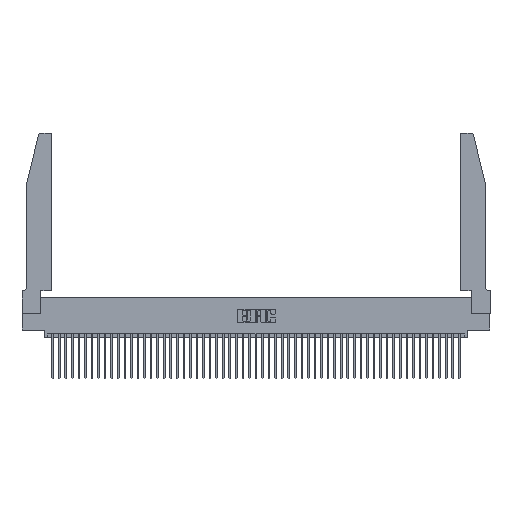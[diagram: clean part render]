
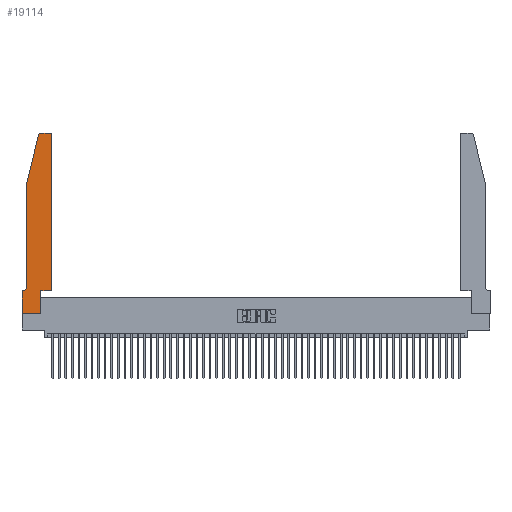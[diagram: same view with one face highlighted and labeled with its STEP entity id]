
A CAD part, top view. The second image highlights one B-rep face of the part: STEP entity #19114.
In plain terms, the highlighted planar face has unit normal (0, 0, 1).
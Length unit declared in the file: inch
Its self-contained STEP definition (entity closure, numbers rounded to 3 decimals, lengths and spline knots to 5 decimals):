
#620 = EDGE_CURVE ( 'NONE', #5873, #29523, #31803, .T. ) ;
#1578 = ORIENTED_EDGE ( 'NONE', *, *, #41890, .T. ) ;
#2566 = VERTEX_POINT ( 'NONE', #39432 ) ;
#3082 = LINE ( 'NONE', #10663, #44157 ) ;
#3701 = CARTESIAN_POINT ( 'NONE',  ( 0.2865, 0.35, 0.37 ) ) ;
#4043 = DIRECTION ( 'NONE',  ( 1., 0., 0. ) ) ;
#4076 = CARTESIAN_POINT ( 'NONE',  ( 0.25487, 2.72718, 0.37 ) ) ;
#4559 = LINE ( 'NONE', #41154, #24607 ) ;
#5214 = DIRECTION ( 'NONE',  ( 0., 0., -1. ) ) ;
#5634 = VERTEX_POINT ( 'NONE', #17853 ) ;
#5873 = VERTEX_POINT ( 'NONE', #9350 ) ;
#6541 = DIRECTION ( 'NONE',  ( 0., -1., 0. ) ) ;
#7667 = VECTOR ( 'NONE', #51362, 39.37008 ) ;
#7882 = DIRECTION ( 'NONE',  ( 0., 1., 0. ) ) ;
#8550 = VERTEX_POINT ( 'NONE', #41912 ) ;
#8673 = LINE ( 'NONE', #29030, #28649 ) ;
#9350 = CARTESIAN_POINT ( 'NONE',  ( 0.0755, 2., 0.37 ) ) ;
#10038 = CARTESIAN_POINT ( 'NONE',  ( 0.4505, 0.35, 0.37 ) ) ;
#10663 = CARTESIAN_POINT ( 'NONE',  ( 0., 0., 0.37 ) ) ;
#10808 = DIRECTION ( 'NONE',  ( 0., -1., 0. ) ) ;
#10912 = EDGE_CURVE ( 'NONE', #2566, #21228, #50021, .T. ) ;
#11011 = CARTESIAN_POINT ( 'NONE',  ( 0.0055, 0.35, 0.37 ) ) ;
#13199 = EDGE_LOOP ( 'NONE', ( #32097, #46073, #20815, #49589, #14871, #13841, #31570, #37342, #35025, #29976, #1578, #30749 ) ) ;
#13446 = CIRCLE ( 'NONE', #44620, 0.03 ) ;
#13841 = ORIENTED_EDGE ( 'NONE', *, *, #39261, .T. ) ;
#13898 = DIRECTION ( 'NONE',  ( 0., 0., 1. ) ) ;
#14679 = CARTESIAN_POINT ( 'NONE',  ( 0.284, 2.75, 0.37 ) ) ;
#14871 = ORIENTED_EDGE ( 'NONE', *, *, #26677, .T. ) ;
#14965 = PLANE ( 'NONE',  #31981 ) ;
#15137 = DIRECTION ( 'NONE',  ( 1., 0., 0. ) ) ;
#15198 = CIRCLE ( 'NONE', #34044, 0.03 ) ;
#17115 = LINE ( 'NONE', #49253, #26450 ) ;
#17155 = VECTOR ( 'NONE', #7882, 39.37008 ) ;
#17853 = CARTESIAN_POINT ( 'NONE',  ( 0.4505, 2.72, 0.37 ) ) ;
#18356 = LINE ( 'NONE', #31590, #7667 ) ;
#18467 = VECTOR ( 'NONE', #6541, 39.37008 ) ;
#19114 = ADVANCED_FACE ( 'NONE', ( #35655 ), #14965, .T. ) ;
#20019 = CARTESIAN_POINT ( 'NONE',  ( 0.4205, 2.75, 0.37 ) ) ;
#20511 = CARTESIAN_POINT ( 'NONE',  ( 0.4205, 2.72, 0.37 ) ) ;
#20815 = ORIENTED_EDGE ( 'NONE', *, *, #32326, .T. ) ;
#21228 = VERTEX_POINT ( 'NONE', #35877 ) ;
#21468 = DIRECTION ( 'NONE',  ( -1., 0., 0. ) ) ;
#22093 = DIRECTION ( 'NONE',  ( 0., 1., 0. ) ) ;
#23004 = VERTEX_POINT ( 'NONE', #11011 ) ;
#23905 = CARTESIAN_POINT ( 'NONE',  ( 0.0755, 0.42, 0.37 ) ) ;
#24022 = VERTEX_POINT ( 'NONE', #4076 ) ;
#24274 = EDGE_CURVE ( 'NONE', #30242, #24022, #13446, .T. ) ;
#24607 = VECTOR ( 'NONE', #21468, 39.37008 ) ;
#26450 = VECTOR ( 'NONE', #29631, 39.37008 ) ;
#26677 = EDGE_CURVE ( 'NONE', #29523, #23004, #49504, .T. ) ;
#26758 = VERTEX_POINT ( 'NONE', #29714 ) ;
#27754 = LINE ( 'NONE', #3701, #17155 ) ;
#28007 = DIRECTION ( 'NONE',  ( 0., 0., 1. ) ) ;
#28286 = EDGE_CURVE ( 'NONE', #8550, #26758, #27754, .T. ) ;
#28649 = VECTOR ( 'NONE', #44893, 39.37008 ) ;
#29030 = CARTESIAN_POINT ( 'NONE',  ( 0.2605, 2.75, 0.37 ) ) ;
#29191 = CARTESIAN_POINT ( 'NONE',  ( 0.0055, 0.42, 0.37 ) ) ;
#29523 = VERTEX_POINT ( 'NONE', #23905 ) ;
#29631 = DIRECTION ( 'NONE',  ( 1., 0., 0. ) ) ;
#29714 = CARTESIAN_POINT ( 'NONE',  ( 0.2865, 0.35, 0.37 ) ) ;
#29976 = ORIENTED_EDGE ( 'NONE', *, *, #48852, .T. ) ;
#30242 = VERTEX_POINT ( 'NONE', #14679 ) ;
#30749 = ORIENTED_EDGE ( 'NONE', *, *, #39676, .T. ) ;
#31570 = ORIENTED_EDGE ( 'NONE', *, *, #10912, .T. ) ;
#31590 = CARTESIAN_POINT ( 'NONE',  ( 0.0755, 2., 0.37 ) ) ;
#31771 = LINE ( 'NONE', #10038, #40962 ) ;
#31803 = LINE ( 'NONE', #46327, #51490 ) ;
#31981 = AXIS2_PLACEMENT_3D ( 'NONE', #34962, #38904, #15137 ) ;
#32097 = ORIENTED_EDGE ( 'NONE', *, *, #41746, .T. ) ;
#32326 = EDGE_CURVE ( 'NONE', #24022, #5873, #18356, .T. ) ;
#32496 = AXIS2_PLACEMENT_3D ( 'NONE', #29191, #5214, #33182 ) ;
#33182 = DIRECTION ( 'NONE',  ( -1., 0., 0. ) ) ;
#33695 = VERTEX_POINT ( 'NONE', #45111 ) ;
#34044 = AXIS2_PLACEMENT_3D ( 'NONE', #20511, #28007, #4043 ) ;
#34502 = DIRECTION ( 'NONE',  ( 1., 0., 0. ) ) ;
#34962 = CARTESIAN_POINT ( 'NONE',  ( 0., 0.35, 0.37 ) ) ;
#35025 = ORIENTED_EDGE ( 'NONE', *, *, #28286, .T. ) ;
#35655 = FACE_OUTER_BOUND ( 'NONE', #13199, .T. ) ;
#35877 = CARTESIAN_POINT ( 'NONE',  ( 0., 0., 0.37 ) ) ;
#37342 = ORIENTED_EDGE ( 'NONE', *, *, #44219, .T. ) ;
#37681 = CARTESIAN_POINT ( 'NONE',  ( 0.284, 2.72, 0.37 ) ) ;
#38904 = DIRECTION ( 'NONE',  ( 0., 0., 1. ) ) ;
#39261 = EDGE_CURVE ( 'NONE', #23004, #2566, #4559, .T. ) ;
#39432 = CARTESIAN_POINT ( 'NONE',  ( 0., 0.35, 0.37 ) ) ;
#39676 = EDGE_CURVE ( 'NONE', #5634, #39680, #15198, .T. ) ;
#39680 = VERTEX_POINT ( 'NONE', #20019 ) ;
#40962 = VECTOR ( 'NONE', #22093, 39.37008 ) ;
#41154 = CARTESIAN_POINT ( 'NONE',  ( 0.0755, 0.35, 0.37 ) ) ;
#41647 = DIRECTION ( 'NONE',  ( 1., 0., 0. ) ) ;
#41746 = EDGE_CURVE ( 'NONE', #39680, #30242, #8673, .T. ) ;
#41890 = EDGE_CURVE ( 'NONE', #33695, #5634, #31771, .T. ) ;
#41912 = CARTESIAN_POINT ( 'NONE',  ( 0.2865, 0., 0.37 ) ) ;
#42224 = CARTESIAN_POINT ( 'NONE',  ( 0., 0., 0.37 ) ) ;
#44157 = VECTOR ( 'NONE', #34502, 39.37008 ) ;
#44219 = EDGE_CURVE ( 'NONE', #21228, #8550, #3082, .T. ) ;
#44620 = AXIS2_PLACEMENT_3D ( 'NONE', #37681, #13898, #41647 ) ;
#44893 = DIRECTION ( 'NONE',  ( -1., 0., 0. ) ) ;
#45111 = CARTESIAN_POINT ( 'NONE',  ( 0.4505, 0.35, 0.37 ) ) ;
#46073 = ORIENTED_EDGE ( 'NONE', *, *, #24274, .T. ) ;
#46327 = CARTESIAN_POINT ( 'NONE',  ( 0.0755, 2., 0.37 ) ) ;
#48852 = EDGE_CURVE ( 'NONE', #26758, #33695, #17115, .T. ) ;
#49253 = CARTESIAN_POINT ( 'NONE',  ( 0.4505, 0.35, 0.37 ) ) ;
#49504 = CIRCLE ( 'NONE', #32496, 0.07 ) ;
#49589 = ORIENTED_EDGE ( 'NONE', *, *, #620, .T. ) ;
#50021 = LINE ( 'NONE', #42224, #18467 ) ;
#51362 = DIRECTION ( 'NONE',  ( -0.239, -0.971, 0. ) ) ;
#51490 = VECTOR ( 'NONE', #10808, 39.37008 ) ;
